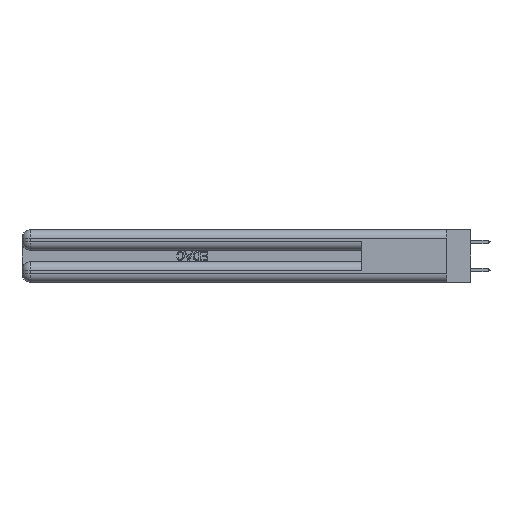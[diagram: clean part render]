
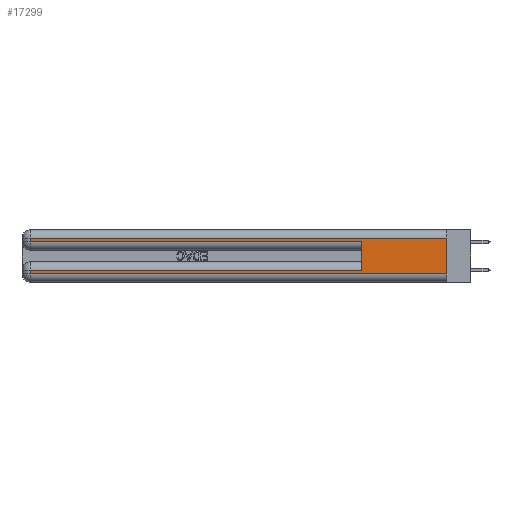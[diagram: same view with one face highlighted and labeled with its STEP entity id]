
A CAD part, left-side view. The second image highlights one B-rep face of the part: STEP entity #17299.
In plain terms, the highlighted planar face has unit normal (-1, 0, 0).
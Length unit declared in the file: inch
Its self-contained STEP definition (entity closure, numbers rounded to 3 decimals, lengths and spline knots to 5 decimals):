
#76 = CARTESIAN_POINT ( 'NONE',  ( 0., 0., 0.06 ) ) ;
#132 = ORIENTED_EDGE ( 'NONE', *, *, #20857, .F. ) ;
#2173 = LINE ( 'NONE', #18465, #28097 ) ;
#4183 = CARTESIAN_POINT ( 'NONE',  ( 0., 0.6, 0.285 ) ) ;
#4637 = PLANE ( 'NONE',  #28888 ) ;
#4735 = DIRECTION ( 'NONE',  ( 0., 0., -1. ) ) ;
#5878 = VERTEX_POINT ( 'NONE', #30841 ) ;
#6679 = DIRECTION ( 'NONE',  ( 0., 1., 0. ) ) ;
#6918 = ORIENTED_EDGE ( 'NONE', *, *, #33731, .T. ) ;
#7022 = DIRECTION ( 'NONE',  ( 0., 0., 1. ) ) ;
#7377 = FACE_OUTER_BOUND ( 'NONE', #18468, .T. ) ;
#7441 = LINE ( 'NONE', #32650, #30583 ) ;
#7606 = CARTESIAN_POINT ( 'NONE',  ( 0., 0., 0.37 ) ) ;
#7788 = VECTOR ( 'NONE', #4735, 39.37008 ) ;
#8915 = ORIENTED_EDGE ( 'NONE', *, *, #16424, .T. ) ;
#9148 = CARTESIAN_POINT ( 'NONE',  ( 0., 2.94, 0.37 ) ) ;
#9864 = CARTESIAN_POINT ( 'NONE',  ( 0., 0.6, 0.145 ) ) ;
#9944 = DIRECTION ( 'NONE',  ( 0., -1., 0. ) ) ;
#12905 = LINE ( 'NONE', #36305, #36497 ) ;
#12969 = ORIENTED_EDGE ( 'NONE', *, *, #27595, .T. ) ;
#13454 = EDGE_CURVE ( 'NONE', #5878, #28050, #33365, .T. ) ;
#13575 = DIRECTION ( 'NONE',  ( 0., 0., -1. ) ) ;
#13636 = VECTOR ( 'NONE', #7022, 39.37008 ) ;
#13671 = VECTOR ( 'NONE', #17420, 39.37008 ) ;
#15539 = LINE ( 'NONE', #32237, #13671 ) ;
#16424 = EDGE_CURVE ( 'NONE', #29438, #29951, #37264, .T. ) ;
#17210 = CARTESIAN_POINT ( 'NONE',  ( 0., 2.94, 0.06 ) ) ;
#17299 = ADVANCED_FACE ( 'NONE', ( #7377 ), #4637, .F. ) ;
#17420 = DIRECTION ( 'NONE',  ( 0., -1., 0. ) ) ;
#17579 = CARTESIAN_POINT ( 'NONE',  ( 0., 0., 0.31 ) ) ;
#17820 = EDGE_CURVE ( 'NONE', #37760, #36714, #30006, .T. ) ;
#18465 = CARTESIAN_POINT ( 'NONE',  ( 0., 0., 0.31 ) ) ;
#18468 = EDGE_LOOP ( 'NONE', ( #18737, #28612, #21704, #19777, #132, #8915, #12969, #6918 ) ) ;
#18737 = ORIENTED_EDGE ( 'NONE', *, *, #17820, .F. ) ;
#19224 = CARTESIAN_POINT ( 'NONE',  ( 0., 2.94, 0.085 ) ) ;
#19777 = ORIENTED_EDGE ( 'NONE', *, *, #20594, .T. ) ;
#20594 = EDGE_CURVE ( 'NONE', #28050, #29845, #15539, .T. ) ;
#20857 = EDGE_CURVE ( 'NONE', #29438, #29845, #29354, .T. ) ;
#21704 = ORIENTED_EDGE ( 'NONE', *, *, #13454, .T. ) ;
#21770 = DIRECTION ( 'NONE',  ( 0., 1., 0. ) ) ;
#22309 = CARTESIAN_POINT ( 'NONE',  ( 0., 0.6, 0.085 ) ) ;
#27595 = EDGE_CURVE ( 'NONE', #29951, #31572, #7441, .T. ) ;
#28050 = VERTEX_POINT ( 'NONE', #31486 ) ;
#28097 = VECTOR ( 'NONE', #6679, 39.37008 ) ;
#28442 = VECTOR ( 'NONE', #21770, 39.37008 ) ;
#28445 = DIRECTION ( 'NONE',  ( 1., 0., 0. ) ) ;
#28612 = ORIENTED_EDGE ( 'NONE', *, *, #34608, .T. ) ;
#28888 = AXIS2_PLACEMENT_3D ( 'NONE', #7606, #28445, #13575 ) ;
#29354 = LINE ( 'NONE', #9864, #13636 ) ;
#29438 = VERTEX_POINT ( 'NONE', #22309 ) ;
#29845 = VERTEX_POINT ( 'NONE', #4183 ) ;
#29951 = VERTEX_POINT ( 'NONE', #19224 ) ;
#30006 = LINE ( 'NONE', #31618, #7788 ) ;
#30583 = VECTOR ( 'NONE', #35639, 39.37008 ) ;
#30841 = CARTESIAN_POINT ( 'NONE',  ( 0., 2.94, 0.31 ) ) ;
#31486 = CARTESIAN_POINT ( 'NONE',  ( 0., 2.94, 0.285 ) ) ;
#31572 = VERTEX_POINT ( 'NONE', #17210 ) ;
#31618 = CARTESIAN_POINT ( 'NONE',  ( 0., 0., 0.37 ) ) ;
#32237 = CARTESIAN_POINT ( 'NONE',  ( 0., 0., 0.285 ) ) ;
#32650 = CARTESIAN_POINT ( 'NONE',  ( 0., 2.94, 0.37 ) ) ;
#33247 = CARTESIAN_POINT ( 'NONE',  ( 0., 0., 0.085 ) ) ;
#33365 = LINE ( 'NONE', #9148, #33808 ) ;
#33731 = EDGE_CURVE ( 'NONE', #31572, #36714, #12905, .T. ) ;
#33808 = VECTOR ( 'NONE', #35776, 39.37008 ) ;
#34608 = EDGE_CURVE ( 'NONE', #37760, #5878, #2173, .T. ) ;
#35639 = DIRECTION ( 'NONE',  ( 0., 0., -1. ) ) ;
#35776 = DIRECTION ( 'NONE',  ( 0., 0., -1. ) ) ;
#36305 = CARTESIAN_POINT ( 'NONE',  ( 0., 0., 0.06 ) ) ;
#36497 = VECTOR ( 'NONE', #9944, 39.37008 ) ;
#36714 = VERTEX_POINT ( 'NONE', #76 ) ;
#37264 = LINE ( 'NONE', #33247, #28442 ) ;
#37760 = VERTEX_POINT ( 'NONE', #17579 ) ;
